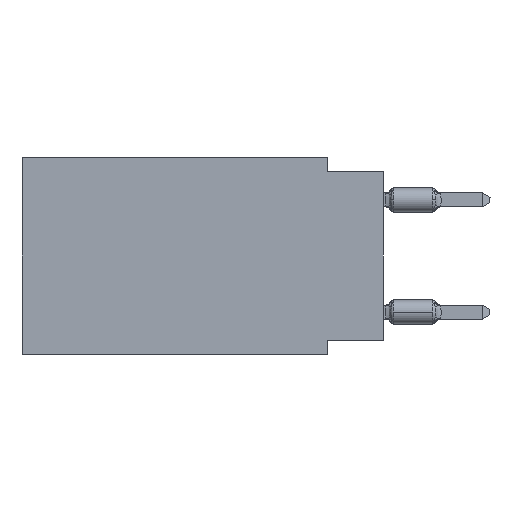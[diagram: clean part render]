
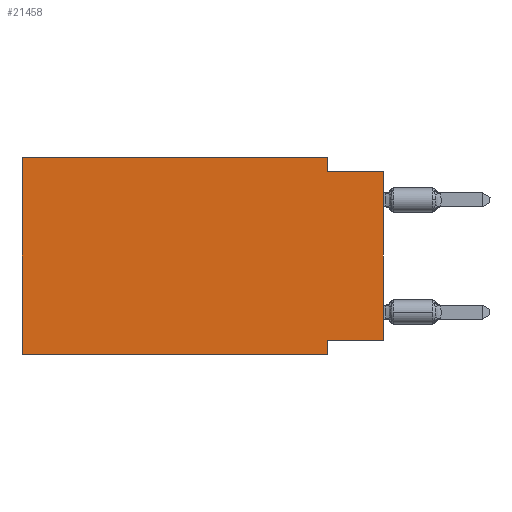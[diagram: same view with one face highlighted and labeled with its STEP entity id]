
A CAD part, left-side view. The second image highlights one B-rep face of the part: STEP entity #21458.
In plain terms, the highlighted planar face has unit normal (-1, 0, 0).
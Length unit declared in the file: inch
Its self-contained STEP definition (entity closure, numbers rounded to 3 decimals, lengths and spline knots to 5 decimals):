
#347 = CARTESIAN_POINT ( 'NONE',  ( 0., 0.1, -0.025 ) ) ;
#1762 = DIRECTION ( 'NONE',  ( 0., 0., -1. ) ) ;
#1779 = VERTEX_POINT ( 'NONE', #40015 ) ;
#2367 = EDGE_CURVE ( 'NONE', #33087, #13023, #34868, .T. ) ;
#2432 = DIRECTION ( 'NONE',  ( 0., 0., 1. ) ) ;
#2763 = VECTOR ( 'NONE', #1762, 39.37008 ) ;
#2777 = EDGE_LOOP ( 'NONE', ( #25352, #18274, #4763, #2809, #26313, #3585, #12977, #18923 ) ) ;
#2809 = ORIENTED_EDGE ( 'NONE', *, *, #12041, .F. ) ;
#3585 = ORIENTED_EDGE ( 'NONE', *, *, #2367, .T. ) ;
#4266 = CARTESIAN_POINT ( 'NONE',  ( 0., 0.645, 0. ) ) ;
#4302 = LINE ( 'NONE', #10498, #5097 ) ;
#4710 = DIRECTION ( 'NONE',  ( 1., 0., 0. ) ) ;
#4713 = VECTOR ( 'NONE', #10227, 39.37008 ) ;
#4763 = ORIENTED_EDGE ( 'NONE', *, *, #19149, .F. ) ;
#5097 = VECTOR ( 'NONE', #7388, 39.37008 ) ;
#5487 = CARTESIAN_POINT ( 'NONE',  ( 0., 0., -0.025 ) ) ;
#6791 = EDGE_CURVE ( 'NONE', #33087, #18707, #37800, .T. ) ;
#7388 = DIRECTION ( 'NONE',  ( 0., -1., 0. ) ) ;
#8637 = DIRECTION ( 'NONE',  ( 0., -1., 0. ) ) ;
#8821 = CARTESIAN_POINT ( 'NONE',  ( 0., 0.1, -0.35 ) ) ;
#9206 = VECTOR ( 'NONE', #2432, 39.37008 ) ;
#9396 = VECTOR ( 'NONE', #26447, 39.37008 ) ;
#9431 = LINE ( 'NONE', #33266, #9396 ) ;
#10227 = DIRECTION ( 'NONE',  ( 0., 0., 1. ) ) ;
#10498 = CARTESIAN_POINT ( 'NONE',  ( 0., 0., -0.025 ) ) ;
#10894 = PLANE ( 'NONE',  #27246 ) ;
#12041 = EDGE_CURVE ( 'NONE', #18707, #12311, #24800, .T. ) ;
#12311 = VERTEX_POINT ( 'NONE', #17005 ) ;
#12977 = ORIENTED_EDGE ( 'NONE', *, *, #31732, .F. ) ;
#13023 = VERTEX_POINT ( 'NONE', #29115 ) ;
#14245 = EDGE_CURVE ( 'NONE', #1779, #18392, #9431, .T. ) ;
#15689 = LINE ( 'NONE', #35314, #9206 ) ;
#17005 = CARTESIAN_POINT ( 'NONE',  ( 0., 0.1, 0. ) ) ;
#17020 = CARTESIAN_POINT ( 'NONE',  ( 0., 0.645, -0.35 ) ) ;
#17719 = CARTESIAN_POINT ( 'NONE',  ( 0., 0.645, 0. ) ) ;
#17734 = VERTEX_POINT ( 'NONE', #347 ) ;
#18274 = ORIENTED_EDGE ( 'NONE', *, *, #38793, .F. ) ;
#18392 = VERTEX_POINT ( 'NONE', #32756 ) ;
#18707 = VERTEX_POINT ( 'NONE', #37556 ) ;
#18923 = ORIENTED_EDGE ( 'NONE', *, *, #14245, .F. ) ;
#19149 = EDGE_CURVE ( 'NONE', #12311, #17734, #32670, .T. ) ;
#20601 = CARTESIAN_POINT ( 'NONE',  ( 0., 0.645, 0. ) ) ;
#21277 = DIRECTION ( 'NONE',  ( 0., 0., -1. ) ) ;
#21458 = ADVANCED_FACE ( 'NONE', ( #27681 ), #10894, .F. ) ;
#22722 = VECTOR ( 'NONE', #30482, 39.37008 ) ;
#23375 = DIRECTION ( 'NONE',  ( 0., 0., -1. ) ) ;
#24800 = LINE ( 'NONE', #17719, #34408 ) ;
#25352 = ORIENTED_EDGE ( 'NONE', *, *, #33527, .T. ) ;
#25634 = LINE ( 'NONE', #8821, #2763 ) ;
#26047 = CARTESIAN_POINT ( 'NONE',  ( 0., 0.1, 0. ) ) ;
#26313 = ORIENTED_EDGE ( 'NONE', *, *, #6791, .F. ) ;
#26447 = DIRECTION ( 'NONE',  ( 0., 1., 0. ) ) ;
#27246 = AXIS2_PLACEMENT_3D ( 'NONE', #4266, #4710, #21277 ) ;
#27681 = FACE_OUTER_BOUND ( 'NONE', #2777, .T. ) ;
#28222 = VERTEX_POINT ( 'NONE', #5487 ) ;
#29115 = CARTESIAN_POINT ( 'NONE',  ( 0., 0.1, -0.35 ) ) ;
#30482 = DIRECTION ( 'NONE',  ( 0., -1., 0. ) ) ;
#31732 = EDGE_CURVE ( 'NONE', #18392, #13023, #25634, .T. ) ;
#32055 = VECTOR ( 'NONE', #23375, 39.37008 ) ;
#32670 = LINE ( 'NONE', #26047, #32055 ) ;
#32756 = CARTESIAN_POINT ( 'NONE',  ( 0., 0.1, -0.325 ) ) ;
#33087 = VERTEX_POINT ( 'NONE', #39542 ) ;
#33266 = CARTESIAN_POINT ( 'NONE',  ( 0., 0., -0.325 ) ) ;
#33527 = EDGE_CURVE ( 'NONE', #1779, #28222, #15689, .T. ) ;
#34408 = VECTOR ( 'NONE', #8637, 39.37008 ) ;
#34868 = LINE ( 'NONE', #17020, #22722 ) ;
#35314 = CARTESIAN_POINT ( 'NONE',  ( 0., 0., 0. ) ) ;
#37556 = CARTESIAN_POINT ( 'NONE',  ( 0., 0.645, 0. ) ) ;
#37800 = LINE ( 'NONE', #20601, #4713 ) ;
#38793 = EDGE_CURVE ( 'NONE', #17734, #28222, #4302, .T. ) ;
#39542 = CARTESIAN_POINT ( 'NONE',  ( 0., 0.645, -0.35 ) ) ;
#40015 = CARTESIAN_POINT ( 'NONE',  ( 0., 0., -0.325 ) ) ;
